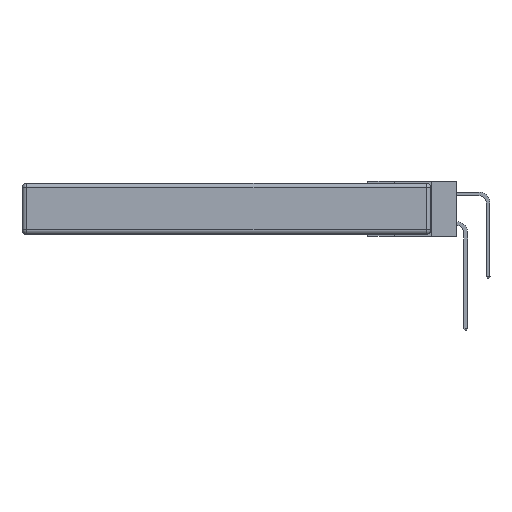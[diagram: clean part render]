
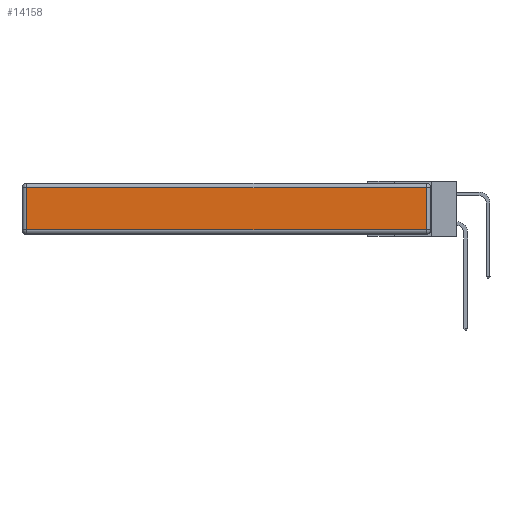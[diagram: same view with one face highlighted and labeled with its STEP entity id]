
A CAD part, left-side view. The second image highlights one B-rep face of the part: STEP entity #14158.
In plain terms, the highlighted planar face has unit normal (-1, 0, 0).
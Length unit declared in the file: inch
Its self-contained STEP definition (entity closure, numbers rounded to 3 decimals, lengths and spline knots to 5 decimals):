
#1137 = ORIENTED_EDGE ( 'NONE', *, *, #25029, .T. ) ;
#1272 = CARTESIAN_POINT ( 'NONE',  ( 0., 2.72, -0.03 ) ) ;
#5686 = VECTOR ( 'NONE', #6864, 39.37008 ) ;
#5895 = CARTESIAN_POINT ( 'NONE',  ( 0., 2.72, -0.313 ) ) ;
#6533 = VECTOR ( 'NONE', #6565, 39.37008 ) ;
#6565 = DIRECTION ( 'NONE',  ( 0., 0., -1. ) ) ;
#6605 = VECTOR ( 'NONE', #8844, 39.37008 ) ;
#6864 = DIRECTION ( 'NONE',  ( 0., -1., 0. ) ) ;
#7248 = CARTESIAN_POINT ( 'NONE',  ( 0., 0., -0.313 ) ) ;
#8624 = EDGE_CURVE ( 'NONE', #12575, #9931, #25848, .T. ) ;
#8844 = DIRECTION ( 'NONE',  ( 0., 1., 0. ) ) ;
#9580 = EDGE_CURVE ( 'NONE', #9931, #23444, #22253, .T. ) ;
#9931 = VERTEX_POINT ( 'NONE', #20799 ) ;
#12269 = CARTESIAN_POINT ( 'NONE',  ( 0., 0.03, -0.343 ) ) ;
#12575 = VERTEX_POINT ( 'NONE', #27519 ) ;
#12659 = DIRECTION ( 'NONE',  ( 0., 0., 1. ) ) ;
#14158 = ADVANCED_FACE ( 'NONE', ( #26519 ), #18279, .T. ) ;
#15334 = EDGE_CURVE ( 'NONE', #23444, #25582, #19093, .T. ) ;
#15522 = ORIENTED_EDGE ( 'NONE', *, *, #15334, .T. ) ;
#15777 = VECTOR ( 'NONE', #12659, 39.37008 ) ;
#17560 = LINE ( 'NONE', #7248, #5686 ) ;
#18279 = PLANE ( 'NONE',  #20796 ) ;
#19093 = LINE ( 'NONE', #26746, #6533 ) ;
#20025 = CARTESIAN_POINT ( 'NONE',  ( 0., 2.75, -0.03 ) ) ;
#20796 = AXIS2_PLACEMENT_3D ( 'NONE', #22436, #25098, #22526 ) ;
#20799 = CARTESIAN_POINT ( 'NONE',  ( 0., 0.03, -0.03 ) ) ;
#22253 = LINE ( 'NONE', #20025, #6605 ) ;
#22436 = CARTESIAN_POINT ( 'NONE',  ( 0., 0., -0.343 ) ) ;
#22526 = DIRECTION ( 'NONE',  ( 0., 0., 1. ) ) ;
#22612 = ORIENTED_EDGE ( 'NONE', *, *, #8624, .T. ) ;
#23444 = VERTEX_POINT ( 'NONE', #1272 ) ;
#25029 = EDGE_CURVE ( 'NONE', #25582, #12575, #17560, .T. ) ;
#25098 = DIRECTION ( 'NONE',  ( -1., 0., 0. ) ) ;
#25582 = VERTEX_POINT ( 'NONE', #5895 ) ;
#25848 = LINE ( 'NONE', #12269, #15777 ) ;
#25876 = ORIENTED_EDGE ( 'NONE', *, *, #9580, .T. ) ;
#26134 = EDGE_LOOP ( 'NONE', ( #1137, #22612, #25876, #15522 ) ) ;
#26519 = FACE_OUTER_BOUND ( 'NONE', #26134, .T. ) ;
#26746 = CARTESIAN_POINT ( 'NONE',  ( 0., 2.72, -0.343 ) ) ;
#27519 = CARTESIAN_POINT ( 'NONE',  ( 0., 0.03, -0.313 ) ) ;
